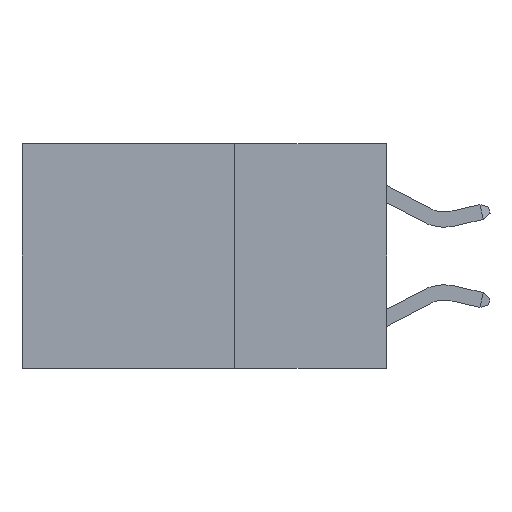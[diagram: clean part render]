
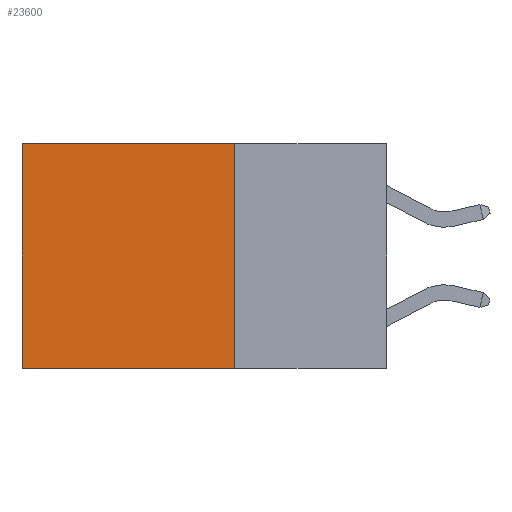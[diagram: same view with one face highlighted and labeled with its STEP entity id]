
A CAD part, left-side view. The second image highlights one B-rep face of the part: STEP entity #23600.
In plain terms, the highlighted planar face has unit normal (-1, 0, 0).
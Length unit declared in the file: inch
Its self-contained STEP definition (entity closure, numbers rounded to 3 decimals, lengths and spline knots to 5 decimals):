
#164 = VERTEX_POINT ( 'NONE', #11342 ) ;
#2591 = EDGE_LOOP ( 'NONE', ( #18124, #21304, #6757, #16402 ) ) ;
#2710 = EDGE_CURVE ( 'NONE', #164, #5464, #5708, .T. ) ;
#4009 = CARTESIAN_POINT ( 'NONE',  ( 0.2625, 0.6, 0. ) ) ;
#4289 = VECTOR ( 'NONE', #9930, 39.37008 ) ;
#4938 = CARTESIAN_POINT ( 'NONE',  ( 0.2625, 0.25, 0. ) ) ;
#4971 = DIRECTION ( 'NONE',  ( 1., 0., 0. ) ) ;
#5412 = VECTOR ( 'NONE', #18558, 39.37008 ) ;
#5464 = VERTEX_POINT ( 'NONE', #10735 ) ;
#5708 = LINE ( 'NONE', #13171, #10017 ) ;
#5832 = VERTEX_POINT ( 'NONE', #13760 ) ;
#6420 = VERTEX_POINT ( 'NONE', #14132 ) ;
#6757 = ORIENTED_EDGE ( 'NONE', *, *, #20991, .F. ) ;
#7484 = VECTOR ( 'NONE', #10419, 39.37008 ) ;
#8042 = LINE ( 'NONE', #4938, #7484 ) ;
#8088 = CARTESIAN_POINT ( 'NONE',  ( 0.2625, 0.25, 0. ) ) ;
#9577 = DIRECTION ( 'NONE',  ( 0., 1., 0. ) ) ;
#9796 = LINE ( 'NONE', #8088, #4289 ) ;
#9930 = DIRECTION ( 'NONE',  ( 0., 0., -1. ) ) ;
#10017 = VECTOR ( 'NONE', #9577, 39.37008 ) ;
#10419 = DIRECTION ( 'NONE',  ( 0., 1., 0. ) ) ;
#10735 = CARTESIAN_POINT ( 'NONE',  ( 0.2625, 0.6, -0.37 ) ) ;
#10856 = LINE ( 'NONE', #4009, #5412 ) ;
#11342 = CARTESIAN_POINT ( 'NONE',  ( 0.2625, 0.25, -0.37 ) ) ;
#13171 = CARTESIAN_POINT ( 'NONE',  ( 0.2625, 0.25, -0.37 ) ) ;
#13760 = CARTESIAN_POINT ( 'NONE',  ( 0.2625, 0.25, 0. ) ) ;
#14132 = CARTESIAN_POINT ( 'NONE',  ( 0.2625, 0.6, 0. ) ) ;
#15838 = PLANE ( 'NONE',  #20503 ) ;
#16402 = ORIENTED_EDGE ( 'NONE', *, *, #18222, .T. ) ;
#17658 = DIRECTION ( 'NONE',  ( 0., 0., -1. ) ) ;
#18124 = ORIENTED_EDGE ( 'NONE', *, *, #22529, .T. ) ;
#18222 = EDGE_CURVE ( 'NONE', #5832, #6420, #8042, .T. ) ;
#18558 = DIRECTION ( 'NONE',  ( 0., 0., -1. ) ) ;
#19232 = FACE_OUTER_BOUND ( 'NONE', #2591, .T. ) ;
#20503 = AXIS2_PLACEMENT_3D ( 'NONE', #21192, #4971, #17658 ) ;
#20991 = EDGE_CURVE ( 'NONE', #5832, #164, #9796, .T. ) ;
#21192 = CARTESIAN_POINT ( 'NONE',  ( 0.2625, 0.25, 0. ) ) ;
#21304 = ORIENTED_EDGE ( 'NONE', *, *, #2710, .F. ) ;
#22529 = EDGE_CURVE ( 'NONE', #6420, #5464, #10856, .T. ) ;
#23600 = ADVANCED_FACE ( 'NONE', ( #19232 ), #15838, .F. ) ;
